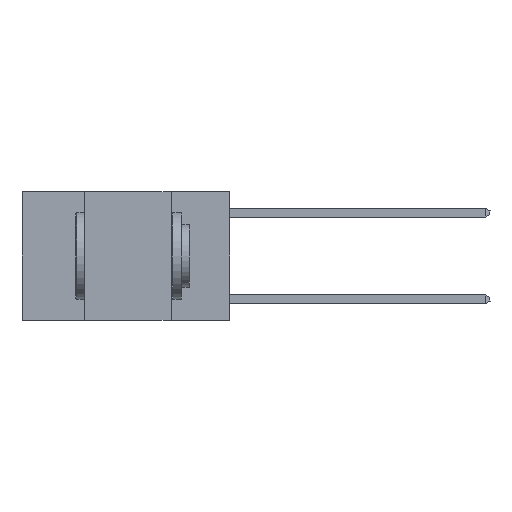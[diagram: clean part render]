
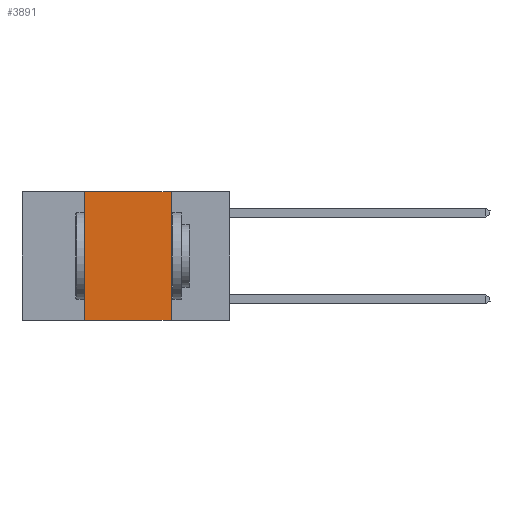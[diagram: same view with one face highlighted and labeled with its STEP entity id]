
A CAD part, left-side view. The second image highlights one B-rep face of the part: STEP entity #3891.
In plain terms, the highlighted planar face has unit normal (-1, 0, 0).
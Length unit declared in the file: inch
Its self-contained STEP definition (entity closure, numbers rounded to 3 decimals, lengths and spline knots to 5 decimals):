
#151 = LINE ( 'NONE', #3539, #4663 ) ;
#2602 = DIRECTION ( 'NONE',  ( 0., 0., 1. ) ) ;
#2997 = CARTESIAN_POINT ( 'NONE',  ( 0., 0.17, 0. ) ) ;
#3074 = CARTESIAN_POINT ( 'NONE',  ( 0., 0.42, 0. ) ) ;
#3430 = ORIENTED_EDGE ( 'NONE', *, *, #12679, .F. ) ;
#3471 = DIRECTION ( 'NONE',  ( 0., -1., 0. ) ) ;
#3539 = CARTESIAN_POINT ( 'NONE',  ( 0., 0.6, -0.37 ) ) ;
#3648 = DIRECTION ( 'NONE',  ( 0., 0., -1. ) ) ;
#3891 = ADVANCED_FACE ( 'NONE', ( #6760 ), #7793, .F. ) ;
#3936 = EDGE_CURVE ( 'NONE', #12554, #9183, #5717, .T. ) ;
#4282 = VECTOR ( 'NONE', #4696, 39.37008 ) ;
#4663 = VECTOR ( 'NONE', #3471, 39.37008 ) ;
#4696 = DIRECTION ( 'NONE',  ( 0., -1., 0. ) ) ;
#5346 = DIRECTION ( 'NONE',  ( 1., 0., 0. ) ) ;
#5352 = CARTESIAN_POINT ( 'NONE',  ( 0., 0.17, -0.37 ) ) ;
#5600 = ORIENTED_EDGE ( 'NONE', *, *, #3936, .F. ) ;
#5688 = CARTESIAN_POINT ( 'NONE',  ( 0., 0.42, -0.37 ) ) ;
#5717 = LINE ( 'NONE', #9914, #4282 ) ;
#5881 = EDGE_CURVE ( 'NONE', #6187, #12554, #11086, .T. ) ;
#6187 = VERTEX_POINT ( 'NONE', #5688 ) ;
#6359 = VERTEX_POINT ( 'NONE', #5352 ) ;
#6441 = ORIENTED_EDGE ( 'NONE', *, *, #5881, .F. ) ;
#6556 = EDGE_CURVE ( 'NONE', #6187, #6359, #151, .T. ) ;
#6760 = FACE_OUTER_BOUND ( 'NONE', #11259, .T. ) ;
#7668 = VECTOR ( 'NONE', #2602, 39.37008 ) ;
#7678 = DIRECTION ( 'NONE',  ( 0., 0., -1. ) ) ;
#7793 = PLANE ( 'NONE',  #9328 ) ;
#7906 = VECTOR ( 'NONE', #7678, 39.37008 ) ;
#8729 = ORIENTED_EDGE ( 'NONE', *, *, #6556, .T. ) ;
#9183 = VERTEX_POINT ( 'NONE', #2997 ) ;
#9328 = AXIS2_PLACEMENT_3D ( 'NONE', #10881, #5346, #3648 ) ;
#9914 = CARTESIAN_POINT ( 'NONE',  ( 0., 0.6, 0. ) ) ;
#10881 = CARTESIAN_POINT ( 'NONE',  ( 0., 0.6, 0. ) ) ;
#11086 = LINE ( 'NONE', #13089, #7668 ) ;
#11259 = EDGE_LOOP ( 'NONE', ( #3430, #5600, #6441, #8729 ) ) ;
#12554 = VERTEX_POINT ( 'NONE', #3074 ) ;
#12679 = EDGE_CURVE ( 'NONE', #9183, #6359, #12983, .T. ) ;
#12983 = LINE ( 'NONE', #13055, #7906 ) ;
#13055 = CARTESIAN_POINT ( 'NONE',  ( 0., 0.17, 0. ) ) ;
#13089 = CARTESIAN_POINT ( 'NONE',  ( 0., 0.42, 0. ) ) ;
